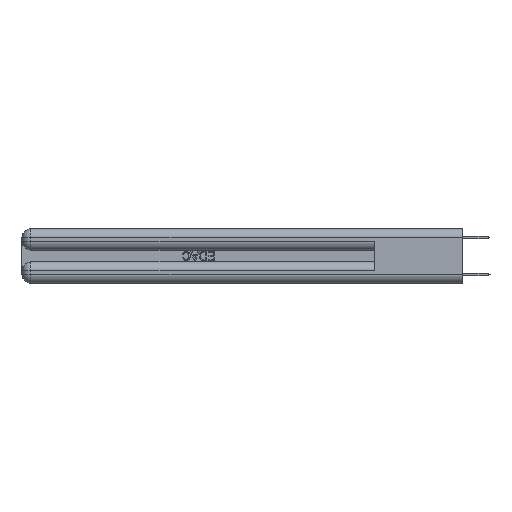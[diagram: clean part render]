
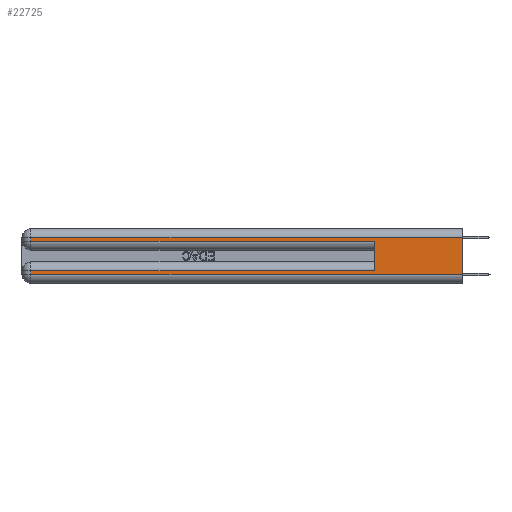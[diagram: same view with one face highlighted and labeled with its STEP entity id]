
A CAD part, left-side view. The second image highlights one B-rep face of the part: STEP entity #22725.
In plain terms, the highlighted planar face has unit normal (-1, 0, 0).
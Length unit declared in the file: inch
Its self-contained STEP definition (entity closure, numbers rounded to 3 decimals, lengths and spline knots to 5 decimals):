
#654 = PLANE ( 'NONE',  #7036 ) ;
#693 = CARTESIAN_POINT ( 'NONE',  ( 0., 0.6, 0.285 ) ) ;
#1119 = DIRECTION ( 'NONE',  ( 0., 0., -1. ) ) ;
#1417 = VERTEX_POINT ( 'NONE', #24458 ) ;
#1967 = VERTEX_POINT ( 'NONE', #23655 ) ;
#2251 = LINE ( 'NONE', #15801, #30410 ) ;
#2676 = VECTOR ( 'NONE', #10760, 39.37008 ) ;
#2975 = EDGE_CURVE ( 'NONE', #34332, #1967, #19344, .T. ) ;
#3521 = VERTEX_POINT ( 'NONE', #26721 ) ;
#3892 = CARTESIAN_POINT ( 'NONE',  ( 0., 0., 0.285 ) ) ;
#4129 = CARTESIAN_POINT ( 'NONE',  ( 0., 0., 0.37 ) ) ;
#4228 = LINE ( 'NONE', #19974, #23329 ) ;
#4527 = DIRECTION ( 'NONE',  ( 0., 0., -1. ) ) ;
#4837 = CARTESIAN_POINT ( 'NONE',  ( 0., 0., 0.06 ) ) ;
#5521 = VECTOR ( 'NONE', #14737, 39.37008 ) ;
#5882 = DIRECTION ( 'NONE',  ( 0., 1., 0. ) ) ;
#6382 = CARTESIAN_POINT ( 'NONE',  ( 0., 2.94, 0.085 ) ) ;
#6823 = LINE ( 'NONE', #4837, #31972 ) ;
#6970 = CARTESIAN_POINT ( 'NONE',  ( 0., 0., 0.37 ) ) ;
#7036 = AXIS2_PLACEMENT_3D ( 'NONE', #4129, #14903, #1119 ) ;
#7427 = EDGE_CURVE ( 'NONE', #1417, #3521, #6823, .T. ) ;
#7688 = EDGE_CURVE ( 'NONE', #1967, #21048, #4228, .T. ) ;
#9835 = EDGE_CURVE ( 'NONE', #34332, #3521, #16668, .T. ) ;
#10645 = VECTOR ( 'NONE', #5882, 39.37008 ) ;
#10760 = DIRECTION ( 'NONE',  ( 0., -1., 0. ) ) ;
#10833 = LINE ( 'NONE', #28125, #32991 ) ;
#11284 = EDGE_CURVE ( 'NONE', #30031, #12499, #10833, .T. ) ;
#11355 = ORIENTED_EDGE ( 'NONE', *, *, #7688, .T. ) ;
#12499 = VERTEX_POINT ( 'NONE', #693 ) ;
#13223 = DIRECTION ( 'NONE',  ( 0., -1., 0. ) ) ;
#14318 = CARTESIAN_POINT ( 'NONE',  ( 0., 2.94, 0.285 ) ) ;
#14480 = CARTESIAN_POINT ( 'NONE',  ( 0., 0., 0.31 ) ) ;
#14737 = DIRECTION ( 'NONE',  ( 0., 1., 0. ) ) ;
#14903 = DIRECTION ( 'NONE',  ( 1., 0., 0. ) ) ;
#15801 = CARTESIAN_POINT ( 'NONE',  ( 0., 2.94, 0.37 ) ) ;
#16405 = VERTEX_POINT ( 'NONE', #6382 ) ;
#16668 = LINE ( 'NONE', #6970, #24454 ) ;
#16738 = DIRECTION ( 'NONE',  ( 0., 0., 1. ) ) ;
#17135 = CARTESIAN_POINT ( 'NONE',  ( 0., 0.6, 0.085 ) ) ;
#17375 = EDGE_CURVE ( 'NONE', #30031, #16405, #19838, .T. ) ;
#19001 = ORIENTED_EDGE ( 'NONE', *, *, #25964, .T. ) ;
#19344 = LINE ( 'NONE', #14480, #10645 ) ;
#19776 = ORIENTED_EDGE ( 'NONE', *, *, #7427, .T. ) ;
#19838 = LINE ( 'NONE', #20206, #5521 ) ;
#19974 = CARTESIAN_POINT ( 'NONE',  ( 0., 2.94, 0.37 ) ) ;
#20038 = DIRECTION ( 'NONE',  ( 0., 0., -1. ) ) ;
#20206 = CARTESIAN_POINT ( 'NONE',  ( 0., 0., 0.085 ) ) ;
#21048 = VERTEX_POINT ( 'NONE', #14318 ) ;
#22725 = ADVANCED_FACE ( 'NONE', ( #25919 ), #654, .F. ) ;
#23329 = VECTOR ( 'NONE', #28364, 39.37008 ) ;
#23655 = CARTESIAN_POINT ( 'NONE',  ( 0., 2.94, 0.31 ) ) ;
#24454 = VECTOR ( 'NONE', #20038, 39.37008 ) ;
#24458 = CARTESIAN_POINT ( 'NONE',  ( 0., 2.94, 0.06 ) ) ;
#25919 = FACE_OUTER_BOUND ( 'NONE', #32070, .T. ) ;
#25964 = EDGE_CURVE ( 'NONE', #21048, #12499, #33902, .T. ) ;
#26012 = ORIENTED_EDGE ( 'NONE', *, *, #17375, .T. ) ;
#26721 = CARTESIAN_POINT ( 'NONE',  ( 0., 0., 0.06 ) ) ;
#28125 = CARTESIAN_POINT ( 'NONE',  ( 0., 0.6, 0.145 ) ) ;
#28364 = DIRECTION ( 'NONE',  ( 0., 0., -1. ) ) ;
#29784 = CARTESIAN_POINT ( 'NONE',  ( 0., 0., 0.31 ) ) ;
#30031 = VERTEX_POINT ( 'NONE', #17135 ) ;
#30410 = VECTOR ( 'NONE', #4527, 39.37008 ) ;
#31403 = ORIENTED_EDGE ( 'NONE', *, *, #35013, .T. ) ;
#31530 = ORIENTED_EDGE ( 'NONE', *, *, #11284, .F. ) ;
#31972 = VECTOR ( 'NONE', #13223, 39.37008 ) ;
#32070 = EDGE_LOOP ( 'NONE', ( #32807, #34702, #11355, #19001, #31530, #26012, #31403, #19776 ) ) ;
#32807 = ORIENTED_EDGE ( 'NONE', *, *, #9835, .F. ) ;
#32991 = VECTOR ( 'NONE', #16738, 39.37008 ) ;
#33902 = LINE ( 'NONE', #3892, #2676 ) ;
#34332 = VERTEX_POINT ( 'NONE', #29784 ) ;
#34702 = ORIENTED_EDGE ( 'NONE', *, *, #2975, .T. ) ;
#35013 = EDGE_CURVE ( 'NONE', #16405, #1417, #2251, .T. ) ;
